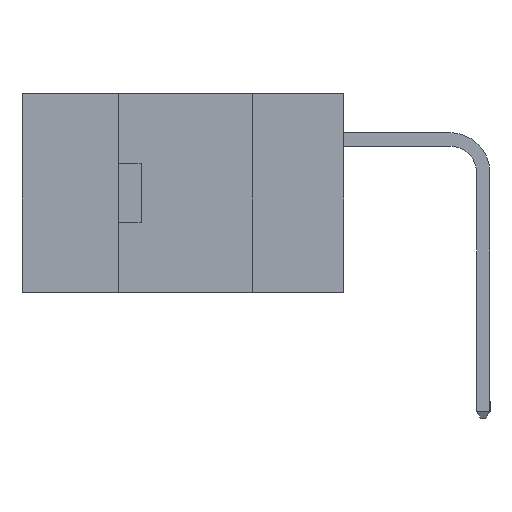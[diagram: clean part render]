
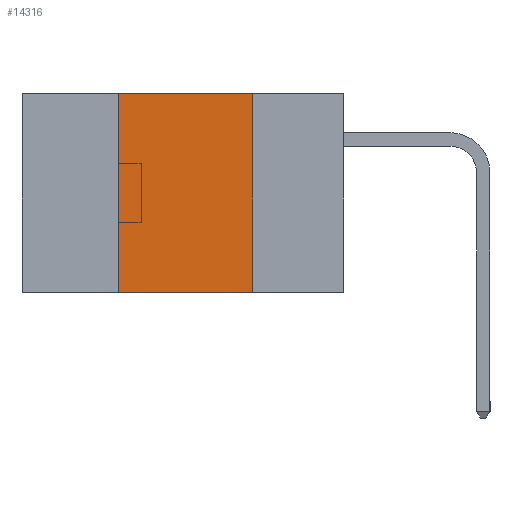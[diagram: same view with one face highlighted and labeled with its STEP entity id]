
A CAD part, left-side view. The second image highlights one B-rep face of the part: STEP entity #14316.
In plain terms, the highlighted planar face has unit normal (-1, 0, 0).
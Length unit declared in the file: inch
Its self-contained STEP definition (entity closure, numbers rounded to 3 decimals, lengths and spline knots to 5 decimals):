
#449 = VERTEX_POINT ( 'NONE', #2492 ) ;
#657 = LINE ( 'NONE', #23267, #7419 ) ;
#2492 = CARTESIAN_POINT ( 'NONE',  ( 0., 0.17, -0.37 ) ) ;
#2523 = VECTOR ( 'NONE', #3523, 39.37008 ) ;
#2660 = VERTEX_POINT ( 'NONE', #16748 ) ;
#2870 = VECTOR ( 'NONE', #8765, 39.37008 ) ;
#3504 = LINE ( 'NONE', #6688, #2870 ) ;
#3523 = DIRECTION ( 'NONE',  ( 0., -1., 0. ) ) ;
#3738 = EDGE_CURVE ( 'NONE', #2660, #15943, #13210, .T. ) ;
#4130 = DIRECTION ( 'NONE',  ( 0., 0., 1. ) ) ;
#5882 = VERTEX_POINT ( 'NONE', #8517 ) ;
#5974 = ORIENTED_EDGE ( 'NONE', *, *, #23258, .F. ) ;
#6653 = DIRECTION ( 'NONE',  ( 0., 0., -1. ) ) ;
#6688 = CARTESIAN_POINT ( 'NONE',  ( 0., 0.6, 0. ) ) ;
#7419 = VECTOR ( 'NONE', #15061, 39.37008 ) ;
#8517 = CARTESIAN_POINT ( 'NONE',  ( 0., 0.17, 0. ) ) ;
#8765 = DIRECTION ( 'NONE',  ( 0., -1., 0. ) ) ;
#8981 = EDGE_LOOP ( 'NONE', ( #5974, #15366, #18971, #20990 ) ) ;
#9604 = AXIS2_PLACEMENT_3D ( 'NONE', #25112, #19000, #6653 ) ;
#10266 = CARTESIAN_POINT ( 'NONE',  ( 0., 0.42, -0.37 ) ) ;
#10339 = CARTESIAN_POINT ( 'NONE',  ( 0., 0.42, 0. ) ) ;
#12392 = EDGE_CURVE ( 'NONE', #15943, #5882, #3504, .T. ) ;
#12941 = FACE_OUTER_BOUND ( 'NONE', #8981, .T. ) ;
#13210 = LINE ( 'NONE', #10266, #23514 ) ;
#14316 = ADVANCED_FACE ( 'NONE', ( #12941 ), #14865, .F. ) ;
#14865 = PLANE ( 'NONE',  #9604 ) ;
#15061 = DIRECTION ( 'NONE',  ( 0., 0., -1. ) ) ;
#15335 = EDGE_CURVE ( 'NONE', #2660, #449, #24447, .T. ) ;
#15366 = ORIENTED_EDGE ( 'NONE', *, *, #12392, .F. ) ;
#15943 = VERTEX_POINT ( 'NONE', #10339 ) ;
#16748 = CARTESIAN_POINT ( 'NONE',  ( 0., 0.42, -0.37 ) ) ;
#17961 = CARTESIAN_POINT ( 'NONE',  ( 0., 0.6, -0.37 ) ) ;
#18971 = ORIENTED_EDGE ( 'NONE', *, *, #3738, .F. ) ;
#19000 = DIRECTION ( 'NONE',  ( 1., 0., 0. ) ) ;
#20990 = ORIENTED_EDGE ( 'NONE', *, *, #15335, .T. ) ;
#23258 = EDGE_CURVE ( 'NONE', #5882, #449, #657, .T. ) ;
#23267 = CARTESIAN_POINT ( 'NONE',  ( 0., 0.17, -0.37 ) ) ;
#23514 = VECTOR ( 'NONE', #4130, 39.37008 ) ;
#24447 = LINE ( 'NONE', #17961, #2523 ) ;
#25112 = CARTESIAN_POINT ( 'NONE',  ( 0., 0.6, 0. ) ) ;
